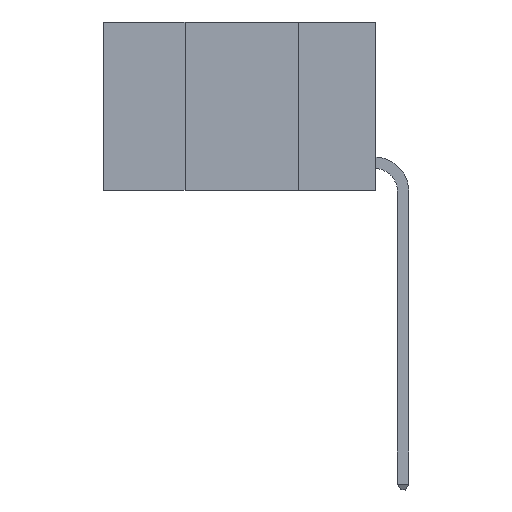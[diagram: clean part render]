
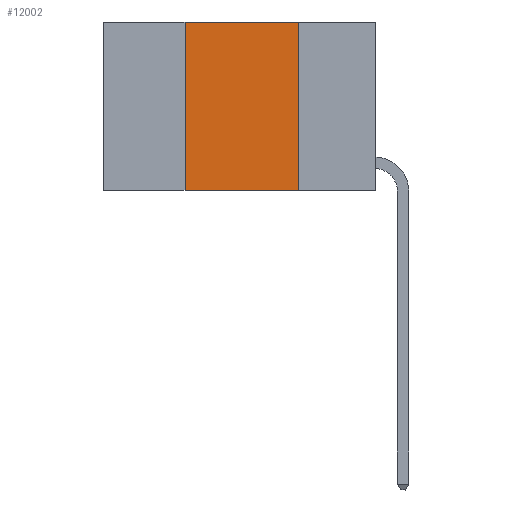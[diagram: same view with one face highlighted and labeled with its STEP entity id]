
A CAD part, left-side view. The second image highlights one B-rep face of the part: STEP entity #12002.
In plain terms, the highlighted planar face has unit normal (-1, 0, 0).
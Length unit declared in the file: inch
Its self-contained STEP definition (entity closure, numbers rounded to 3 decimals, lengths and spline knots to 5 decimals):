
#310 = CARTESIAN_POINT ( 'NONE',  ( 0., 0.6, 0. ) ) ;
#437 = VERTEX_POINT ( 'NONE', #10202 ) ;
#1020 = CARTESIAN_POINT ( 'NONE',  ( 0., 0.6, -0.37 ) ) ;
#1403 = FACE_OUTER_BOUND ( 'NONE', #12852, .T. ) ;
#1579 = CARTESIAN_POINT ( 'NONE',  ( 0., 0.17, 0. ) ) ;
#2073 = CARTESIAN_POINT ( 'NONE',  ( 0., 0.17, 0. ) ) ;
#2489 = CARTESIAN_POINT ( 'NONE',  ( 0., 0.42, -0.37 ) ) ;
#3987 = CARTESIAN_POINT ( 'NONE',  ( 0., 0.42, 0. ) ) ;
#4509 = DIRECTION ( 'NONE',  ( 0., -1., 0. ) ) ;
#4916 = VECTOR ( 'NONE', #16683, 39.37008 ) ;
#5106 = ORIENTED_EDGE ( 'NONE', *, *, #10746, .F. ) ;
#5372 = EDGE_CURVE ( 'NONE', #8119, #9026, #12465, .T. ) ;
#5387 = DIRECTION ( 'NONE',  ( 0., 0., 1. ) ) ;
#5845 = DIRECTION ( 'NONE',  ( 1., 0., 0. ) ) ;
#5853 = CARTESIAN_POINT ( 'NONE',  ( 0., 0.6, 0. ) ) ;
#5880 = LINE ( 'NONE', #1579, #12618 ) ;
#6375 = LINE ( 'NONE', #3987, #16691 ) ;
#8119 = VERTEX_POINT ( 'NONE', #2489 ) ;
#8864 = VECTOR ( 'NONE', #4509, 39.37008 ) ;
#9026 = VERTEX_POINT ( 'NONE', #9435 ) ;
#9435 = CARTESIAN_POINT ( 'NONE',  ( 0., 0.17, -0.37 ) ) ;
#9770 = AXIS2_PLACEMENT_3D ( 'NONE', #310, #5845, #15261 ) ;
#9796 = EDGE_CURVE ( 'NONE', #437, #14044, #12068, .T. ) ;
#10202 = CARTESIAN_POINT ( 'NONE',  ( 0., 0.42, 0. ) ) ;
#10746 = EDGE_CURVE ( 'NONE', #8119, #437, #6375, .T. ) ;
#12002 = ADVANCED_FACE ( 'NONE', ( #1403 ), #13846, .F. ) ;
#12068 = LINE ( 'NONE', #5853, #4916 ) ;
#12465 = LINE ( 'NONE', #1020, #8864 ) ;
#12618 = VECTOR ( 'NONE', #16521, 39.37008 ) ;
#12708 = ORIENTED_EDGE ( 'NONE', *, *, #9796, .F. ) ;
#12852 = EDGE_LOOP ( 'NONE', ( #16296, #12708, #5106, #15456 ) ) ;
#13325 = EDGE_CURVE ( 'NONE', #14044, #9026, #5880, .T. ) ;
#13846 = PLANE ( 'NONE',  #9770 ) ;
#14044 = VERTEX_POINT ( 'NONE', #2073 ) ;
#15261 = DIRECTION ( 'NONE',  ( 0., 0., -1. ) ) ;
#15456 = ORIENTED_EDGE ( 'NONE', *, *, #5372, .T. ) ;
#16296 = ORIENTED_EDGE ( 'NONE', *, *, #13325, .F. ) ;
#16521 = DIRECTION ( 'NONE',  ( 0., 0., -1. ) ) ;
#16683 = DIRECTION ( 'NONE',  ( 0., -1., 0. ) ) ;
#16691 = VECTOR ( 'NONE', #5387, 39.37008 ) ;
